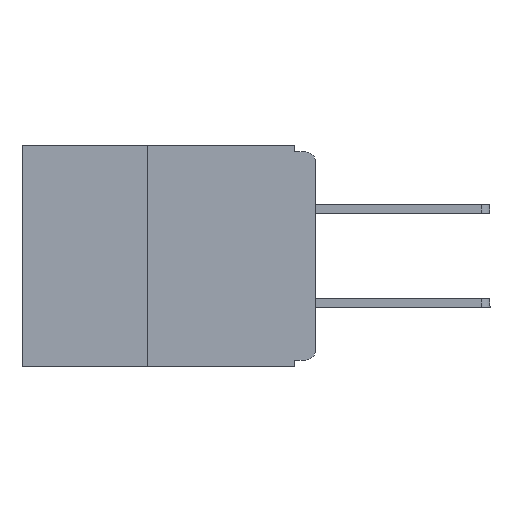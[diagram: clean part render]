
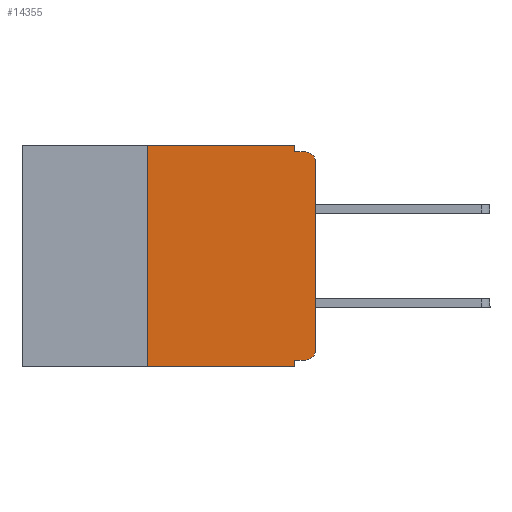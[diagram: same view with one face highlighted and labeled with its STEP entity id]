
A CAD part, left-side view. The second image highlights one B-rep face of the part: STEP entity #14355.
In plain terms, the highlighted planar face has unit normal (-1, 0, 0).
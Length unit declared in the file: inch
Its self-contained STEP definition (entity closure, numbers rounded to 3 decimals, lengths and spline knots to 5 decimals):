
#174 = CARTESIAN_POINT ( 'NONE',  ( 0., 0.437, 0. ) ) ;
#745 = EDGE_CURVE ( 'NONE', #11195, #6959, #4843, .T. ) ;
#873 = CARTESIAN_POINT ( 'NONE',  ( 0., 0.25, -0.33 ) ) ;
#1689 = LINE ( 'NONE', #9952, #7059 ) ;
#1912 = CARTESIAN_POINT ( 'NONE',  ( 0., 0.031, -0.33 ) ) ;
#2214 = DIRECTION ( 'NONE',  ( 0., -1., 0. ) ) ;
#2388 = LINE ( 'NONE', #25021, #25208 ) ;
#3070 = LINE ( 'NONE', #17840, #19407 ) ;
#3303 = VECTOR ( 'NONE', #27557, 39.37008 ) ;
#4084 = ORIENTED_EDGE ( 'NONE', *, *, #23766, .F. ) ;
#4250 = VERTEX_POINT ( 'NONE', #13626 ) ;
#4843 = LINE ( 'NONE', #174, #16725 ) ;
#5101 = VERTEX_POINT ( 'NONE', #25373 ) ;
#5895 = DIRECTION ( 'NONE',  ( -1., 0., 0. ) ) ;
#6065 = DIRECTION ( 'NONE',  ( 1., 0., 0. ) ) ;
#6332 = EDGE_CURVE ( 'NONE', #4250, #11195, #26713, .T. ) ;
#6959 = VERTEX_POINT ( 'NONE', #23279 ) ;
#7059 = VECTOR ( 'NONE', #18838, 39.37008 ) ;
#7563 = ORIENTED_EDGE ( 'NONE', *, *, #12846, .T. ) ;
#7703 = CIRCLE ( 'NONE', #22920, 0.015 ) ;
#8138 = CARTESIAN_POINT ( 'NONE',  ( 0., 0.015, -0.01 ) ) ;
#8257 = VECTOR ( 'NONE', #8965, 39.37008 ) ;
#8590 = VECTOR ( 'NONE', #11796, 39.37008 ) ;
#8612 = VERTEX_POINT ( 'NONE', #14176 ) ;
#8965 = DIRECTION ( 'NONE',  ( 0., 0., -1. ) ) ;
#9316 = LINE ( 'NONE', #27020, #8590 ) ;
#9712 = DIRECTION ( 'NONE',  ( 0., 0., -1. ) ) ;
#9803 = DIRECTION ( 'NONE',  ( -1., 0., 0. ) ) ;
#9952 = CARTESIAN_POINT ( 'NONE',  ( 0., 0., -0.32 ) ) ;
#10694 = CARTESIAN_POINT ( 'NONE',  ( 0., 0.25, 0. ) ) ;
#11076 = ORIENTED_EDGE ( 'NONE', *, *, #22465, .F. ) ;
#11195 = VERTEX_POINT ( 'NONE', #10694 ) ;
#11570 = VERTEX_POINT ( 'NONE', #20838 ) ;
#11796 = DIRECTION ( 'NONE',  ( 0., 0., 1. ) ) ;
#12361 = CARTESIAN_POINT ( 'NONE',  ( 0., 0.031, -0.32 ) ) ;
#12485 = ORIENTED_EDGE ( 'NONE', *, *, #745, .F. ) ;
#12553 = VECTOR ( 'NONE', #27283, 39.37008 ) ;
#12694 = CARTESIAN_POINT ( 'NONE',  ( 0., 0.437, 0. ) ) ;
#12846 = EDGE_CURVE ( 'NONE', #25700, #13031, #23550, .T. ) ;
#12858 = ORIENTED_EDGE ( 'NONE', *, *, #22696, .T. ) ;
#13031 = VERTEX_POINT ( 'NONE', #8138 ) ;
#13133 = FACE_OUTER_BOUND ( 'NONE', #23514, .T. ) ;
#13626 = CARTESIAN_POINT ( 'NONE',  ( 0., 0.25, -0.33 ) ) ;
#14176 = CARTESIAN_POINT ( 'NONE',  ( 0., 0.031, -0.01 ) ) ;
#14355 = ADVANCED_FACE ( 'NONE', ( #13133 ), #19284, .F. ) ;
#14908 = VERTEX_POINT ( 'NONE', #12361 ) ;
#16650 = ORIENTED_EDGE ( 'NONE', *, *, #6332, .F. ) ;
#16725 = VECTOR ( 'NONE', #22165, 39.37008 ) ;
#17840 = CARTESIAN_POINT ( 'NONE',  ( 0., 0., -0.01 ) ) ;
#17978 = ORIENTED_EDGE ( 'NONE', *, *, #21708, .T. ) ;
#18084 = AXIS2_PLACEMENT_3D ( 'NONE', #12694, #6065, #21445 ) ;
#18838 = DIRECTION ( 'NONE',  ( 0., 1., 0. ) ) ;
#19067 = LINE ( 'NONE', #20759, #12553 ) ;
#19128 = CARTESIAN_POINT ( 'NONE',  ( 0., 0.015, -0.305 ) ) ;
#19284 = PLANE ( 'NONE',  #18084 ) ;
#19407 = VECTOR ( 'NONE', #2214, 39.37008 ) ;
#20638 = VERTEX_POINT ( 'NONE', #1912 ) ;
#20759 = CARTESIAN_POINT ( 'NONE',  ( 0., 0.437, -0.33 ) ) ;
#20838 = CARTESIAN_POINT ( 'NONE',  ( 0., 0.015, -0.32 ) ) ;
#20926 = EDGE_CURVE ( 'NONE', #6959, #8612, #2388, .T. ) ;
#21283 = DIRECTION ( 'NONE',  ( 0., 0., -1. ) ) ;
#21445 = DIRECTION ( 'NONE',  ( 0., 0., -1. ) ) ;
#21708 = EDGE_CURVE ( 'NONE', #11570, #5101, #7703, .T. ) ;
#22165 = DIRECTION ( 'NONE',  ( 0., -1., 0. ) ) ;
#22225 = AXIS2_PLACEMENT_3D ( 'NONE', #22938, #9803, #25119 ) ;
#22465 = EDGE_CURVE ( 'NONE', #8612, #13031, #3070, .T. ) ;
#22694 = ORIENTED_EDGE ( 'NONE', *, *, #20926, .F. ) ;
#22696 = EDGE_CURVE ( 'NONE', #4250, #20638, #19067, .T. ) ;
#22920 = AXIS2_PLACEMENT_3D ( 'NONE', #19128, #5895, #21283 ) ;
#22938 = CARTESIAN_POINT ( 'NONE',  ( 0., 0.015, -0.025 ) ) ;
#23024 = ORIENTED_EDGE ( 'NONE', *, *, #23936, .T. ) ;
#23279 = CARTESIAN_POINT ( 'NONE',  ( 0., 0.031, 0. ) ) ;
#23514 = EDGE_LOOP ( 'NONE', ( #23024, #7563, #11076, #22694, #12485, #16650, #12858, #4084, #25123, #17978 ) ) ;
#23550 = CIRCLE ( 'NONE', #22225, 0.015 ) ;
#23766 = EDGE_CURVE ( 'NONE', #14908, #20638, #24380, .T. ) ;
#23936 = EDGE_CURVE ( 'NONE', #5101, #25700, #9316, .T. ) ;
#24380 = LINE ( 'NONE', #28562, #8257 ) ;
#25021 = CARTESIAN_POINT ( 'NONE',  ( 0., 0.031, 0. ) ) ;
#25119 = DIRECTION ( 'NONE',  ( 0., 0., -1. ) ) ;
#25123 = ORIENTED_EDGE ( 'NONE', *, *, #28462, .F. ) ;
#25208 = VECTOR ( 'NONE', #9712, 39.37008 ) ;
#25373 = CARTESIAN_POINT ( 'NONE',  ( 0., 0., -0.305 ) ) ;
#25700 = VERTEX_POINT ( 'NONE', #27962 ) ;
#26713 = LINE ( 'NONE', #873, #3303 ) ;
#27020 = CARTESIAN_POINT ( 'NONE',  ( 0., 0., 0. ) ) ;
#27283 = DIRECTION ( 'NONE',  ( 0., -1., 0. ) ) ;
#27557 = DIRECTION ( 'NONE',  ( 0., 0., 1. ) ) ;
#27962 = CARTESIAN_POINT ( 'NONE',  ( 0., 0., -0.025 ) ) ;
#28462 = EDGE_CURVE ( 'NONE', #11570, #14908, #1689, .T. ) ;
#28562 = CARTESIAN_POINT ( 'NONE',  ( 0., 0.031, -0.33 ) ) ;
